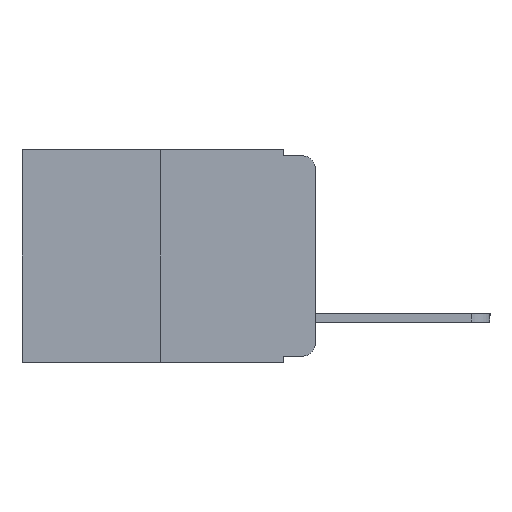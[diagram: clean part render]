
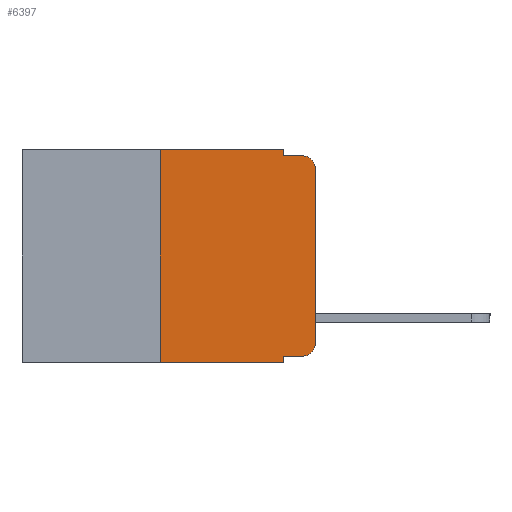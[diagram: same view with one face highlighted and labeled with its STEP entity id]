
A CAD part, left-side view. The second image highlights one B-rep face of the part: STEP entity #6397.
In plain terms, the highlighted planar face has unit normal (-1, 0, 0).
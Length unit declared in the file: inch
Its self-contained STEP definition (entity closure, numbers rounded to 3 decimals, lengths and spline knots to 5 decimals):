
#286 = EDGE_CURVE ( 'NONE', #7054, #14301, #12233, .T. ) ;
#294 = VECTOR ( 'NONE', #7454, 39.37008 ) ;
#830 = ORIENTED_EDGE ( 'NONE', *, *, #10340, .F. ) ;
#964 = VECTOR ( 'NONE', #4254, 39.37008 ) ;
#1130 = LINE ( 'NONE', #8592, #11276 ) ;
#1256 = CARTESIAN_POINT ( 'NONE',  ( 0., 0.051, 0. ) ) ;
#1510 = CARTESIAN_POINT ( 'NONE',  ( 0., 0.473, -0.343 ) ) ;
#1580 = VERTEX_POINT ( 'NONE', #9618 ) ;
#2464 = LINE ( 'NONE', #6449, #17205 ) ;
#2478 = VECTOR ( 'NONE', #2498, 39.37008 ) ;
#2498 = DIRECTION ( 'NONE',  ( 0., 0., 1. ) ) ;
#2592 = EDGE_CURVE ( 'NONE', #1580, #9622, #1130, .T. ) ;
#3026 = AXIS2_PLACEMENT_3D ( 'NONE', #14969, #6411, #16348 ) ;
#3243 = EDGE_CURVE ( 'NONE', #16831, #11483, #4255, .T. ) ;
#3610 = VERTEX_POINT ( 'NONE', #7594 ) ;
#3834 = CARTESIAN_POINT ( 'NONE',  ( 0., 0.473, 0. ) ) ;
#4159 = LINE ( 'NONE', #8835, #294 ) ;
#4197 = DIRECTION ( 'NONE',  ( 0., -1., 0. ) ) ;
#4254 = DIRECTION ( 'NONE',  ( 0., 0., -1. ) ) ;
#4255 = LINE ( 'NONE', #3834, #16093 ) ;
#4381 = DIRECTION ( 'NONE',  ( -1., 0., 0. ) ) ;
#4402 = DIRECTION ( 'NONE',  ( 0., -1., 0. ) ) ;
#4596 = CIRCLE ( 'NONE', #3026, 0.02 ) ;
#4699 = ORIENTED_EDGE ( 'NONE', *, *, #11150, .T. ) ;
#4856 = VERTEX_POINT ( 'NONE', #8996 ) ;
#5277 = DIRECTION ( 'NONE',  ( 0., -1., 0. ) ) ;
#5990 = EDGE_CURVE ( 'NONE', #9622, #17551, #11843, .T. ) ;
#6306 = LINE ( 'NONE', #18199, #2478 ) ;
#6339 = EDGE_LOOP ( 'NONE', ( #11204, #13388, #830, #6474, #16497, #10332, #15439, #13001, #14319, #4699 ) ) ;
#6397 = ADVANCED_FACE ( 'NONE', ( #8004 ), #14131, .F. ) ;
#6411 = DIRECTION ( 'NONE',  ( -1., 0., 0. ) ) ;
#6449 = CARTESIAN_POINT ( 'NONE',  ( 0., 0.051, 0. ) ) ;
#6474 = ORIENTED_EDGE ( 'NONE', *, *, #13655, .F. ) ;
#7054 = VERTEX_POINT ( 'NONE', #18596 ) ;
#7087 = CARTESIAN_POINT ( 'NONE',  ( 0., 0.473, 0. ) ) ;
#7454 = DIRECTION ( 'NONE',  ( 0., -1., 0. ) ) ;
#7594 = CARTESIAN_POINT ( 'NONE',  ( 0., 0.25, -0.343 ) ) ;
#8004 = FACE_OUTER_BOUND ( 'NONE', #6339, .T. ) ;
#8388 = DIRECTION ( 'NONE',  ( 0., 0., 1. ) ) ;
#8531 = DIRECTION ( 'NONE',  ( 0., 0., -1. ) ) ;
#8592 = CARTESIAN_POINT ( 'NONE',  ( 0., 0., 0. ) ) ;
#8656 = VECTOR ( 'NONE', #4402, 39.37008 ) ;
#8671 = CARTESIAN_POINT ( 'NONE',  ( 0., 0., -0.03 ) ) ;
#8835 = CARTESIAN_POINT ( 'NONE',  ( 0., 0.051, -0.01 ) ) ;
#8913 = CARTESIAN_POINT ( 'NONE',  ( 0., 0.02, -0.01 ) ) ;
#8996 = CARTESIAN_POINT ( 'NONE',  ( 0., 0.051, -0.343 ) ) ;
#9618 = CARTESIAN_POINT ( 'NONE',  ( 0., 0., -0.313 ) ) ;
#9622 = VERTEX_POINT ( 'NONE', #8671 ) ;
#9876 = AXIS2_PLACEMENT_3D ( 'NONE', #7087, #17037, #8531 ) ;
#10332 = ORIENTED_EDGE ( 'NONE', *, *, #13218, .F. ) ;
#10340 = EDGE_CURVE ( 'NONE', #10637, #17551, #4159, .T. ) ;
#10637 = VERTEX_POINT ( 'NONE', #13796 ) ;
#10917 = EDGE_CURVE ( 'NONE', #3610, #4856, #16198, .T. ) ;
#11150 = EDGE_CURVE ( 'NONE', #14301, #1580, #4596, .T. ) ;
#11204 = ORIENTED_EDGE ( 'NONE', *, *, #2592, .T. ) ;
#11276 = VECTOR ( 'NONE', #8388, 39.37008 ) ;
#11483 = VERTEX_POINT ( 'NONE', #1256 ) ;
#11843 = CIRCLE ( 'NONE', #13415, 0.02 ) ;
#12233 = LINE ( 'NONE', #17678, #15989 ) ;
#12973 = CARTESIAN_POINT ( 'NONE',  ( 0., 0.02, -0.03 ) ) ;
#13001 = ORIENTED_EDGE ( 'NONE', *, *, #17427, .F. ) ;
#13218 = EDGE_CURVE ( 'NONE', #3610, #16831, #6306, .T. ) ;
#13388 = ORIENTED_EDGE ( 'NONE', *, *, #5990, .T. ) ;
#13415 = AXIS2_PLACEMENT_3D ( 'NONE', #12973, #4381, #14398 ) ;
#13563 = DIRECTION ( 'NONE',  ( 0., 0., -1. ) ) ;
#13655 = EDGE_CURVE ( 'NONE', #11483, #10637, #2464, .T. ) ;
#13796 = CARTESIAN_POINT ( 'NONE',  ( 0., 0.051, -0.01 ) ) ;
#14131 = PLANE ( 'NONE',  #9876 ) ;
#14301 = VERTEX_POINT ( 'NONE', #15547 ) ;
#14319 = ORIENTED_EDGE ( 'NONE', *, *, #286, .T. ) ;
#14398 = DIRECTION ( 'NONE',  ( 0., 0., -1. ) ) ;
#14969 = CARTESIAN_POINT ( 'NONE',  ( 0., 0.02, -0.313 ) ) ;
#15315 = LINE ( 'NONE', #17106, #964 ) ;
#15439 = ORIENTED_EDGE ( 'NONE', *, *, #10917, .T. ) ;
#15547 = CARTESIAN_POINT ( 'NONE',  ( 0., 0.02, -0.333 ) ) ;
#15989 = VECTOR ( 'NONE', #4197, 39.37008 ) ;
#16093 = VECTOR ( 'NONE', #5277, 39.37008 ) ;
#16198 = LINE ( 'NONE', #1510, #8656 ) ;
#16348 = DIRECTION ( 'NONE',  ( 0., 0., -1. ) ) ;
#16497 = ORIENTED_EDGE ( 'NONE', *, *, #3243, .F. ) ;
#16831 = VERTEX_POINT ( 'NONE', #17295 ) ;
#17037 = DIRECTION ( 'NONE',  ( 1., 0., 0. ) ) ;
#17106 = CARTESIAN_POINT ( 'NONE',  ( 0., 0.051, 0. ) ) ;
#17205 = VECTOR ( 'NONE', #13563, 39.37008 ) ;
#17295 = CARTESIAN_POINT ( 'NONE',  ( 0., 0.25, 0. ) ) ;
#17427 = EDGE_CURVE ( 'NONE', #7054, #4856, #15315, .T. ) ;
#17551 = VERTEX_POINT ( 'NONE', #8913 ) ;
#17678 = CARTESIAN_POINT ( 'NONE',  ( 0., 0.051, -0.333 ) ) ;
#18199 = CARTESIAN_POINT ( 'NONE',  ( 0., 0.25, 0. ) ) ;
#18596 = CARTESIAN_POINT ( 'NONE',  ( 0., 0.051, -0.333 ) ) ;
